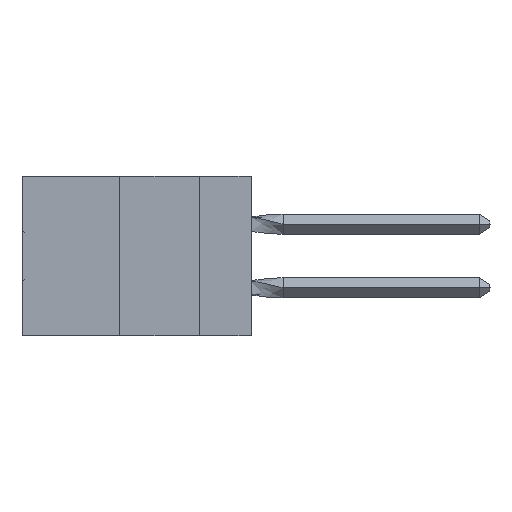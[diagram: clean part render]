
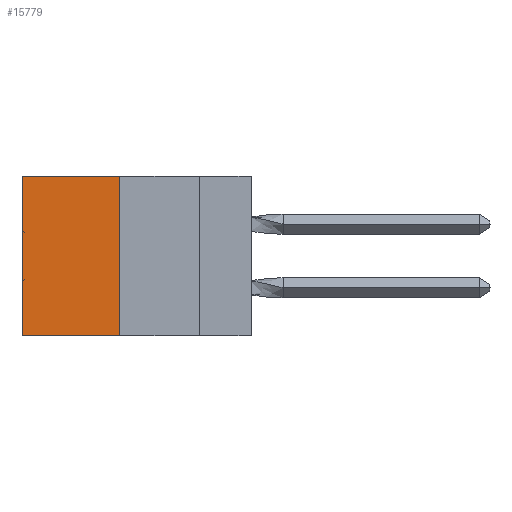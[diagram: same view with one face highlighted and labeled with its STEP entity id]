
A CAD part, left-side view. The second image highlights one B-rep face of the part: STEP entity #15779.
In plain terms, the highlighted planar face has unit normal (-1, 0, 0).
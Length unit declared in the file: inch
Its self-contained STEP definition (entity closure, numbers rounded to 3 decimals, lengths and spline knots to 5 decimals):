
#242 = DIRECTION ( 'NONE',  ( 0., 1., 0. ) ) ;
#568 = VERTEX_POINT ( 'NONE', #49234 ) ;
#2216 = EDGE_CURVE ( 'NONE', #4116, #23884, #26441, .T. ) ;
#4116 = VERTEX_POINT ( 'NONE', #14973 ) ;
#5305 = CARTESIAN_POINT ( 'NONE',  ( 0.305, 0.413, -0.5 ) ) ;
#6036 = DIRECTION ( 'NONE',  ( 0., 0., -1. ) ) ;
#6648 = DIRECTION ( 'NONE',  ( 0., 0., -1. ) ) ;
#8214 = VECTOR ( 'NONE', #242, 39.37008 ) ;
#8446 = CARTESIAN_POINT ( 'NONE',  ( 0.305, 0.72, -0.5 ) ) ;
#9351 = DIRECTION ( 'NONE',  ( 0., 0., -1. ) ) ;
#9538 = CARTESIAN_POINT ( 'NONE',  ( 0.305, 0.413, -0.5 ) ) ;
#13081 = VERTEX_POINT ( 'NONE', #40520 ) ;
#13942 = DIRECTION ( 'NONE',  ( 1., 0., 0. ) ) ;
#14973 = CARTESIAN_POINT ( 'NONE',  ( 0.305, 0.72, 0. ) ) ;
#15100 = AXIS2_PLACEMENT_3D ( 'NONE', #9538, #13942, #9351 ) ;
#15779 = ADVANCED_FACE ( 'NONE', ( #27061 ), #38889, .F. ) ;
#17666 = EDGE_LOOP ( 'NONE', ( #20757, #45646, #39845, #48207 ) ) ;
#20757 = ORIENTED_EDGE ( 'NONE', *, *, #2216, .T. ) ;
#22084 = LINE ( 'NONE', #22649, #52934 ) ;
#22649 = CARTESIAN_POINT ( 'NONE',  ( 0.305, 0.413, 0. ) ) ;
#23884 = VERTEX_POINT ( 'NONE', #8446 ) ;
#26441 = LINE ( 'NONE', #35972, #28378 ) ;
#27061 = FACE_OUTER_BOUND ( 'NONE', #17666, .T. ) ;
#28378 = VECTOR ( 'NONE', #6648, 39.37008 ) ;
#30076 = VECTOR ( 'NONE', #6036, 39.37008 ) ;
#30167 = EDGE_CURVE ( 'NONE', #13081, #23884, #44357, .T. ) ;
#35972 = CARTESIAN_POINT ( 'NONE',  ( 0.305, 0.72, -0.5 ) ) ;
#38889 = PLANE ( 'NONE',  #15100 ) ;
#39845 = ORIENTED_EDGE ( 'NONE', *, *, #45690, .F. ) ;
#40111 = DIRECTION ( 'NONE',  ( 0., 1., 0. ) ) ;
#40520 = CARTESIAN_POINT ( 'NONE',  ( 0.305, 0.413, -0.5 ) ) ;
#44357 = LINE ( 'NONE', #50542, #8214 ) ;
#45646 = ORIENTED_EDGE ( 'NONE', *, *, #30167, .F. ) ;
#45690 = EDGE_CURVE ( 'NONE', #568, #13081, #54354, .T. ) ;
#48207 = ORIENTED_EDGE ( 'NONE', *, *, #52020, .T. ) ;
#49234 = CARTESIAN_POINT ( 'NONE',  ( 0.305, 0.413, 0. ) ) ;
#50542 = CARTESIAN_POINT ( 'NONE',  ( 0.305, 0.413, -0.5 ) ) ;
#52020 = EDGE_CURVE ( 'NONE', #568, #4116, #22084, .T. ) ;
#52934 = VECTOR ( 'NONE', #40111, 39.37008 ) ;
#54354 = LINE ( 'NONE', #5305, #30076 ) ;
